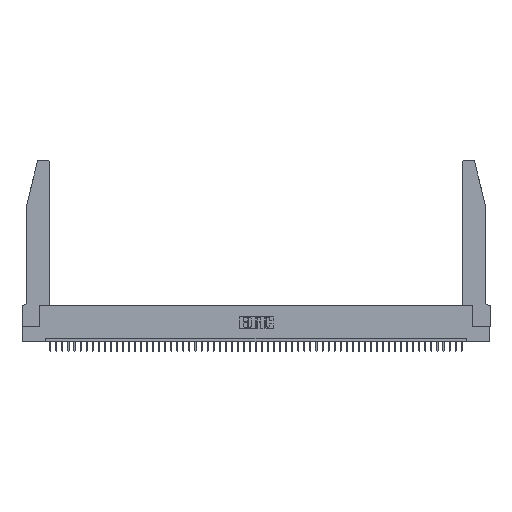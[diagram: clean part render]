
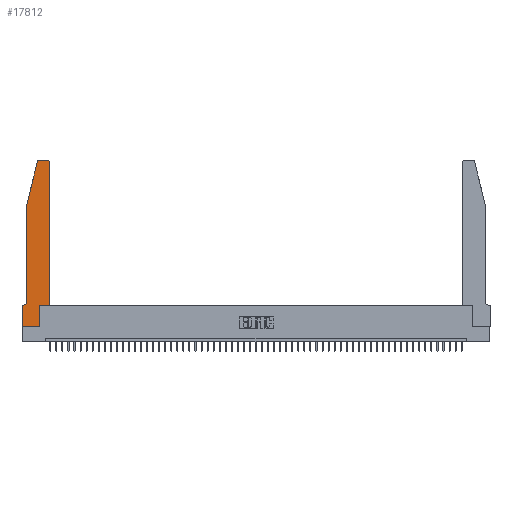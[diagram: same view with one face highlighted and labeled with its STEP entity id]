
A CAD part, top view. The second image highlights one B-rep face of the part: STEP entity #17812.
In plain terms, the highlighted planar face has unit normal (0, 0, 1).
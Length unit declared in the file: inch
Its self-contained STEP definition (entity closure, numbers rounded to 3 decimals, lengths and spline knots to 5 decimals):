
#151 = DIRECTION ( 'NONE',  ( 0., 1., 0. ) ) ;
#413 = EDGE_LOOP ( 'NONE', ( #19148, #35273, #48619, #30547, #1377, #32403, #2585, #24273, #38791, #3431, #11844, #9189 ) ) ;
#759 = EDGE_CURVE ( 'NONE', #9719, #38806, #20126, .T. ) ;
#766 = DIRECTION ( 'NONE',  ( 0., -1., 0. ) ) ;
#1377 = ORIENTED_EDGE ( 'NONE', *, *, #52303, .T. ) ;
#2166 = DIRECTION ( 'NONE',  ( 0., 0., 1. ) ) ;
#2515 = LINE ( 'NONE', #6977, #3189 ) ;
#2585 = ORIENTED_EDGE ( 'NONE', *, *, #37141, .T. ) ;
#3189 = VECTOR ( 'NONE', #10546, 39.37008 ) ;
#3431 = ORIENTED_EDGE ( 'NONE', *, *, #51257, .T. ) ;
#4098 = VECTOR ( 'NONE', #18679, 39.37008 ) ;
#4373 = CARTESIAN_POINT ( 'NONE',  ( 0.4505, 0.35, 0.37 ) ) ;
#5658 = LINE ( 'NONE', #39904, #37108 ) ;
#5933 = CARTESIAN_POINT ( 'NONE',  ( 0.0755, 2., 0.37 ) ) ;
#6608 = VECTOR ( 'NONE', #13514, 39.37008 ) ;
#6977 = CARTESIAN_POINT ( 'NONE',  ( 0.0755, 2., 0.37 ) ) ;
#8039 = LINE ( 'NONE', #9129, #50347 ) ;
#8235 = EDGE_CURVE ( 'NONE', #19132, #13167, #36433, .T. ) ;
#8749 = LINE ( 'NONE', #14634, #18351 ) ;
#9033 = CIRCLE ( 'NONE', #50092, 0.07 ) ;
#9129 = CARTESIAN_POINT ( 'NONE',  ( 0., 0., 0.37 ) ) ;
#9135 = EDGE_CURVE ( 'NONE', #20397, #19132, #8749, .T. ) ;
#9189 = ORIENTED_EDGE ( 'NONE', *, *, #49804, .T. ) ;
#9282 = VERTEX_POINT ( 'NONE', #21233 ) ;
#9719 = VERTEX_POINT ( 'NONE', #21062 ) ;
#10546 = DIRECTION ( 'NONE',  ( -0.239, -0.971, 0. ) ) ;
#11844 = ORIENTED_EDGE ( 'NONE', *, *, #23128, .T. ) ;
#11938 = DIRECTION ( 'NONE',  ( -1., 0., 0. ) ) ;
#12399 = CARTESIAN_POINT ( 'NONE',  ( 0.2865, 0., 0.37 ) ) ;
#13167 = VERTEX_POINT ( 'NONE', #48696 ) ;
#13514 = DIRECTION ( 'NONE',  ( -1., 0., 0. ) ) ;
#14155 = DIRECTION ( 'NONE',  ( 1., 0., 0. ) ) ;
#14244 = VECTOR ( 'NONE', #45442, 39.37008 ) ;
#14634 = CARTESIAN_POINT ( 'NONE',  ( 0.2605, 2.75, 0.37 ) ) ;
#14988 = DIRECTION ( 'NONE',  ( 0., 1., 0. ) ) ;
#15407 = VECTOR ( 'NONE', #14988, 39.37008 ) ;
#16210 = LINE ( 'NONE', #37402, #6608 ) ;
#16554 = DIRECTION ( 'NONE',  ( 0., 0., -1. ) ) ;
#17303 = DIRECTION ( 'NONE',  ( 1., 0., 0. ) ) ;
#17388 = LINE ( 'NONE', #31490, #15407 ) ;
#17655 = PLANE ( 'NONE',  #42325 ) ;
#17812 = ADVANCED_FACE ( 'NONE', ( #18220 ), #17655, .T. ) ;
#18220 = FACE_OUTER_BOUND ( 'NONE', #413, .T. ) ;
#18351 = VECTOR ( 'NONE', #11938, 39.37008 ) ;
#18679 = DIRECTION ( 'NONE',  ( 1., 0., 0. ) ) ;
#18825 = DIRECTION ( 'NONE',  ( 0., 0., 1. ) ) ;
#19132 = VERTEX_POINT ( 'NONE', #48318 ) ;
#19148 = ORIENTED_EDGE ( 'NONE', *, *, #9135, .T. ) ;
#19182 = DIRECTION ( 'NONE',  ( 1., 0., 0. ) ) ;
#19793 = AXIS2_PLACEMENT_3D ( 'NONE', #39281, #2166, #14155 ) ;
#20126 = LINE ( 'NONE', #43439, #4098 ) ;
#20160 = CARTESIAN_POINT ( 'NONE',  ( 0.0755, 0.42, 0.37 ) ) ;
#20329 = CARTESIAN_POINT ( 'NONE',  ( 0.0055, 0.42, 0.37 ) ) ;
#20397 = VERTEX_POINT ( 'NONE', #36653 ) ;
#21062 = CARTESIAN_POINT ( 'NONE',  ( 0., 0., 0.37 ) ) ;
#21074 = CARTESIAN_POINT ( 'NONE',  ( 0.4505, 0.35, 0.37 ) ) ;
#21163 = VERTEX_POINT ( 'NONE', #21325 ) ;
#21233 = CARTESIAN_POINT ( 'NONE',  ( 0.2865, 0.35, 0.37 ) ) ;
#21307 = EDGE_CURVE ( 'NONE', #13167, #36123, #2515, .T. ) ;
#21325 = CARTESIAN_POINT ( 'NONE',  ( 0.4505, 2.72, 0.37 ) ) ;
#22888 = VERTEX_POINT ( 'NONE', #52124 ) ;
#22961 = CARTESIAN_POINT ( 'NONE',  ( 0.284, 2.72, 0.37 ) ) ;
#23128 = EDGE_CURVE ( 'NONE', #48227, #21163, #29238, .T. ) ;
#23153 = AXIS2_PLACEMENT_3D ( 'NONE', #22961, #18825, #19182 ) ;
#24273 = ORIENTED_EDGE ( 'NONE', *, *, #759, .T. ) ;
#25724 = EDGE_CURVE ( 'NONE', #38806, #9282, #17388, .T. ) ;
#28342 = EDGE_CURVE ( 'NONE', #36123, #33388, #5658, .T. ) ;
#28728 = CARTESIAN_POINT ( 'NONE',  ( 0.4505, 0.35, 0.37 ) ) ;
#28775 = DIRECTION ( 'NONE',  ( -1., 0., 0. ) ) ;
#29238 = LINE ( 'NONE', #21074, #31177 ) ;
#30547 = ORIENTED_EDGE ( 'NONE', *, *, #28342, .T. ) ;
#31177 = VECTOR ( 'NONE', #151, 39.37008 ) ;
#31490 = CARTESIAN_POINT ( 'NONE',  ( 0.2865, 0.35, 0.37 ) ) ;
#32403 = ORIENTED_EDGE ( 'NONE', *, *, #50849, .T. ) ;
#33388 = VERTEX_POINT ( 'NONE', #20160 ) ;
#35273 = ORIENTED_EDGE ( 'NONE', *, *, #8235, .T. ) ;
#35742 = DIRECTION ( 'NONE',  ( 0., -1., 0. ) ) ;
#36123 = VERTEX_POINT ( 'NONE', #5933 ) ;
#36433 = CIRCLE ( 'NONE', #23153, 0.03 ) ;
#36653 = CARTESIAN_POINT ( 'NONE',  ( 0.4205, 2.75, 0.37 ) ) ;
#36820 = VERTEX_POINT ( 'NONE', #48427 ) ;
#37108 = VECTOR ( 'NONE', #35742, 39.37008 ) ;
#37141 = EDGE_CURVE ( 'NONE', #22888, #9719, #8039, .T. ) ;
#37402 = CARTESIAN_POINT ( 'NONE',  ( 0.0755, 0.35, 0.37 ) ) ;
#38791 = ORIENTED_EDGE ( 'NONE', *, *, #25724, .T. ) ;
#38806 = VERTEX_POINT ( 'NONE', #12399 ) ;
#39281 = CARTESIAN_POINT ( 'NONE',  ( 0.4205, 2.72, 0.37 ) ) ;
#39904 = CARTESIAN_POINT ( 'NONE',  ( 0.0755, 2., 0.37 ) ) ;
#42325 = AXIS2_PLACEMENT_3D ( 'NONE', #45666, #46376, #17303 ) ;
#43439 = CARTESIAN_POINT ( 'NONE',  ( 0., 0., 0.37 ) ) ;
#45442 = DIRECTION ( 'NONE',  ( 1., 0., 0. ) ) ;
#45666 = CARTESIAN_POINT ( 'NONE',  ( 0., 0.35, 0.37 ) ) ;
#46376 = DIRECTION ( 'NONE',  ( 0., 0., 1. ) ) ;
#48227 = VERTEX_POINT ( 'NONE', #28728 ) ;
#48318 = CARTESIAN_POINT ( 'NONE',  ( 0.284, 2.75, 0.37 ) ) ;
#48427 = CARTESIAN_POINT ( 'NONE',  ( 0.0055, 0.35, 0.37 ) ) ;
#48619 = ORIENTED_EDGE ( 'NONE', *, *, #21307, .T. ) ;
#48696 = CARTESIAN_POINT ( 'NONE',  ( 0.25487, 2.72718, 0.37 ) ) ;
#49804 = EDGE_CURVE ( 'NONE', #21163, #20397, #51628, .T. ) ;
#50092 = AXIS2_PLACEMENT_3D ( 'NONE', #20329, #16554, #28775 ) ;
#50347 = VECTOR ( 'NONE', #766, 39.37008 ) ;
#50849 = EDGE_CURVE ( 'NONE', #36820, #22888, #16210, .T. ) ;
#51257 = EDGE_CURVE ( 'NONE', #9282, #48227, #51468, .T. ) ;
#51468 = LINE ( 'NONE', #4373, #14244 ) ;
#51628 = CIRCLE ( 'NONE', #19793, 0.03 ) ;
#52124 = CARTESIAN_POINT ( 'NONE',  ( 0., 0.35, 0.37 ) ) ;
#52303 = EDGE_CURVE ( 'NONE', #33388, #36820, #9033, .T. ) ;
